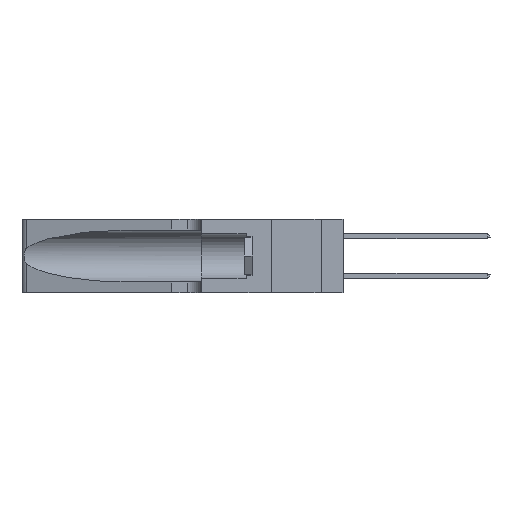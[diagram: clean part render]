
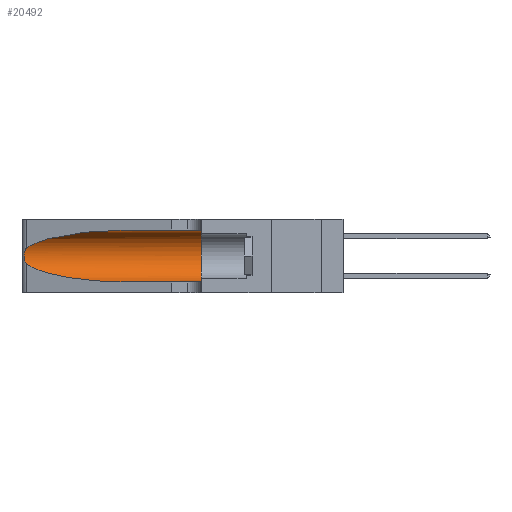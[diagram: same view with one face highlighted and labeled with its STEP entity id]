
A CAD part, left-side view. The second image highlights one B-rep face of the part: STEP entity #20492.
In plain terms, the highlighted cylindrical face has radius 3.308 mm (diameter 6.617 mm), a partial arc.
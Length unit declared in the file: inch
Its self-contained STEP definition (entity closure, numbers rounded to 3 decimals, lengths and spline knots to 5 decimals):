
#1252 = CARTESIAN_POINT ( 'NONE',  ( 0.18966, 0.96281, 0.31525 ) ) ;
#1335 = VECTOR ( 'NONE', #17612, 39.37008 ) ;
#1499 = CARTESIAN_POINT ( 'NONE',  ( 0.1305, 0.72297, 0.05475 ) ) ;
#1993 = ORIENTED_EDGE ( 'NONE', *, *, #23549, .T. ) ;
#2426 = LINE ( 'NONE', #10965, #29862 ) ;
#2625 = CARTESIAN_POINT ( 'NONE',  ( 0.26075, 1.23896, 0.19203 ) ) ;
#2832 = EDGE_CURVE ( 'NONE', #13639, #13827, #8521, .T. ) ;
#3325 = FACE_OUTER_BOUND ( 'NONE', #26445, .T. ) ;
#3971 = CARTESIAN_POINT ( 'NONE',  ( 0.2373, 1.15595, 0.28018 ) ) ;
#4594 = CARTESIAN_POINT ( 'NONE',  ( 0.1305, 0.72297, 0.05475 ) ) ;
#5333 = CARTESIAN_POINT ( 'NONE',  ( 0.26017, 1.23833, 0.17102 ) ) ;
#7098 = VERTEX_POINT ( 'NONE', #25647 ) ;
#8048 = CARTESIAN_POINT ( 'NONE',  ( 0.25789, 1.23486, 0.15765 ) ) ;
#8521 = LINE ( 'NONE', #17507, #1335 ) ;
#9216 = ORIENTED_EDGE ( 'NONE', *, *, #18942, .T. ) ;
#9385 = CARTESIAN_POINT ( 'NONE',  ( 0.25487, 1.22718, 0.14631 ) ) ;
#10488 = B_SPLINE_CURVE_WITH_KNOTS ( 'NONE', 3,
 ( #31766, #13261, #13146, #15938, #34414, #18597, #2625, #21258, #5333, #23944, #8048, #26578, #10694, #29246 ),
 .UNSPECIFIED., .F., .F.,
 ( 4, 2, 2, 2, 2, 2, 4 ),
 ( 0., 0.00027, 0.00053, 0.00107, 0.0016, 0.00187, 0.00214 ),
 .UNSPECIFIED. ) ;
#10694 = CARTESIAN_POINT ( 'NONE',  ( 0.25555, 1.22993, 0.14849 ) ) ;
#10965 = CARTESIAN_POINT ( 'NONE',  ( 0.1305, 1.61858, 0.05475 ) ) ;
#12538 = DIRECTION ( 'NONE',  ( 0., 1., 0. ) ) ;
#12546 = CARTESIAN_POINT ( 'NONE',  ( 0.1305, 1.61858, 0.185 ) ) ;
#13146 = CARTESIAN_POINT ( 'NONE',  ( 0.25639, 1.23184, 0.21858 ) ) ;
#13261 = CARTESIAN_POINT ( 'NONE',  ( 0.25555, 1.22994, 0.2215 ) ) ;
#13639 = VERTEX_POINT ( 'NONE', #19561 ) ;
#13827 = VERTEX_POINT ( 'NONE', #33529 ) ;
#14102 =( BOUNDED_CURVE ( )  B_SPLINE_CURVE ( 3, ( #17266, #1252, #3971, #22592 ),
 .UNSPECIFIED., .F., .F. ) 
 B_SPLINE_CURVE_WITH_KNOTS ( ( 4, 4 ),
 ( 1.5708, 2.84003 ),
 .UNSPECIFIED. ) 
 CURVE ( )  GEOMETRIC_REPRESENTATION_ITEM ( )  RATIONAL_B_SPLINE_CURVE ( ( 1., 0.87, 0.87, 1. ) ) 
 REPRESENTATION_ITEM ( '' )  );
#14127 = CIRCLE ( 'NONE', #21202, 0.13025 ) ;
#14393 = ORIENTED_EDGE ( 'NONE', *, *, #2832, .F. ) ;
#14816 = CARTESIAN_POINT ( 'NONE',  ( 0.25487, 1.22718, 0.22369 ) ) ;
#15099 = EDGE_CURVE ( 'NONE', #13827, #7098, #14127, .T. ) ;
#15125 = VERTEX_POINT ( 'NONE', #4594 ) ;
#15207 = DIRECTION ( 'NONE',  ( 0., 0., -1. ) ) ;
#15938 = CARTESIAN_POINT ( 'NONE',  ( 0.25787, 1.23484, 0.2124 ) ) ;
#16511 = EDGE_CURVE ( 'NONE', #17574, #20673, #10488, .T. ) ;
#16683 = CYLINDRICAL_SURFACE ( 'NONE', #28396, 0.13025 ) ;
#17266 = CARTESIAN_POINT ( 'NONE',  ( 0.1305, 0.72297, 0.31525 ) ) ;
#17507 = CARTESIAN_POINT ( 'NONE',  ( 0.1305, 1.61858, 0.31525 ) ) ;
#17510 = CARTESIAN_POINT ( 'NONE',  ( 0.18966, 0.96281, 0.05475 ) ) ;
#17574 = VERTEX_POINT ( 'NONE', #14816 ) ;
#17612 = DIRECTION ( 'NONE',  ( 0., -1., 0. ) ) ;
#18597 = CARTESIAN_POINT ( 'NONE',  ( 0.26018, 1.23835, 0.19895 ) ) ;
#18942 = EDGE_CURVE ( 'NONE', #20673, #15125, #26439, .T. ) ;
#19561 = CARTESIAN_POINT ( 'NONE',  ( 0.1305, 0.72297, 0.31525 ) ) ;
#20219 = ORIENTED_EDGE ( 'NONE', *, *, #31880, .T. ) ;
#20492 = ADVANCED_FACE ( 'NONE', ( #3325 ), #16683, .F. ) ;
#20673 = VERTEX_POINT ( 'NONE', #23789 ) ;
#21202 = AXIS2_PLACEMENT_3D ( 'NONE', #28389, #12538, #31040 ) ;
#21258 = CARTESIAN_POINT ( 'NONE',  ( 0.26075, 1.23896, 0.178 ) ) ;
#21629 = DIRECTION ( 'NONE',  ( 0., -1., 0. ) ) ;
#22592 = CARTESIAN_POINT ( 'NONE',  ( 0.25487, 1.22718, 0.22369 ) ) ;
#23549 = EDGE_CURVE ( 'NONE', #13639, #17574, #14102, .T. ) ;
#23789 = CARTESIAN_POINT ( 'NONE',  ( 0.25487, 1.22718, 0.14631 ) ) ;
#23944 = CARTESIAN_POINT ( 'NONE',  ( 0.25856, 1.23593, 0.16098 ) ) ;
#25647 = CARTESIAN_POINT ( 'NONE',  ( 0.1305, 0.35, 0.05475 ) ) ;
#26439 =( BOUNDED_CURVE ( )  B_SPLINE_CURVE ( 3, ( #9385, #33230, #17510, #1499 ),
 .UNSPECIFIED., .F., .T. ) 
 B_SPLINE_CURVE_WITH_KNOTS ( ( 4, 4 ),
 ( 3.44316, 4.71239 ),
 .UNSPECIFIED. ) 
 CURVE ( )  GEOMETRIC_REPRESENTATION_ITEM ( )  RATIONAL_B_SPLINE_CURVE ( ( 1., 0.87, 0.87, 1. ) ) 
 REPRESENTATION_ITEM ( '' )  );
#26445 = EDGE_LOOP ( 'NONE', ( #1993, #32606, #9216, #20219, #33134, #14393 ) ) ;
#26578 = CARTESIAN_POINT ( 'NONE',  ( 0.25639, 1.23186, 0.15144 ) ) ;
#28389 = CARTESIAN_POINT ( 'NONE',  ( 0.1305, 0.35, 0.185 ) ) ;
#28396 = AXIS2_PLACEMENT_3D ( 'NONE', #12546, #31050, #15207 ) ;
#29246 = CARTESIAN_POINT ( 'NONE',  ( 0.25487, 1.22718, 0.14631 ) ) ;
#29862 = VECTOR ( 'NONE', #21629, 39.37008 ) ;
#31040 = DIRECTION ( 'NONE',  ( 0., 0., 1. ) ) ;
#31050 = DIRECTION ( 'NONE',  ( 0., -1., 0. ) ) ;
#31766 = CARTESIAN_POINT ( 'NONE',  ( 0.25487, 1.22718, 0.22369 ) ) ;
#31880 = EDGE_CURVE ( 'NONE', #15125, #7098, #2426, .T. ) ;
#32606 = ORIENTED_EDGE ( 'NONE', *, *, #16511, .T. ) ;
#33134 = ORIENTED_EDGE ( 'NONE', *, *, #15099, .F. ) ;
#33230 = CARTESIAN_POINT ( 'NONE',  ( 0.2373, 1.15595, 0.08982 ) ) ;
#33529 = CARTESIAN_POINT ( 'NONE',  ( 0.1305, 0.35, 0.31525 ) ) ;
#34414 = CARTESIAN_POINT ( 'NONE',  ( 0.25854, 1.2359, 0.20912 ) ) ;
